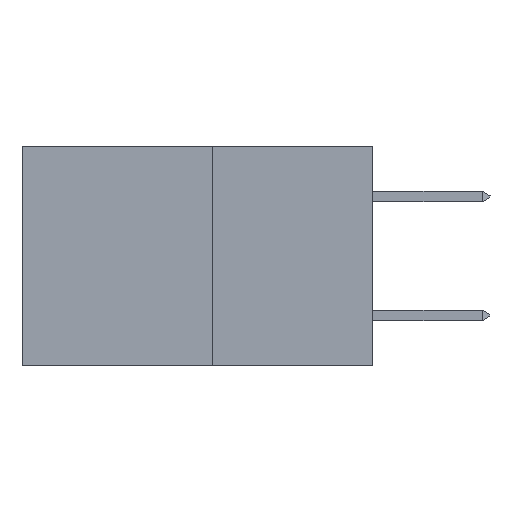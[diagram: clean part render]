
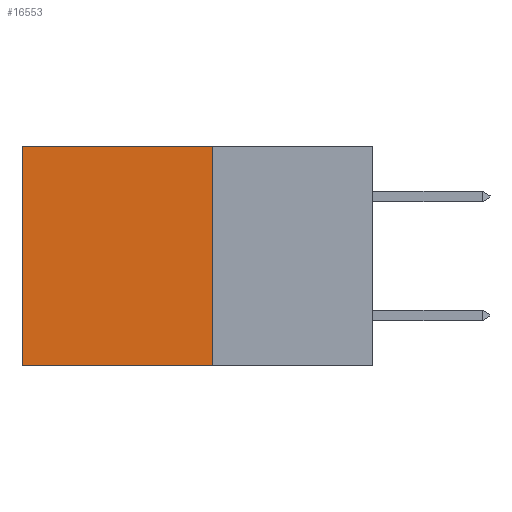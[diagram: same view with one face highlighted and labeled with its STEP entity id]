
A CAD part, left-side view. The second image highlights one B-rep face of the part: STEP entity #16553.
In plain terms, the highlighted planar face has unit normal (-1, 0, 0).
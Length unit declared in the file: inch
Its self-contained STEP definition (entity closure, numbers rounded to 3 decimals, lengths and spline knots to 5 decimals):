
#2171 = CARTESIAN_POINT ( 'NONE',  ( 0.277, 0.27, 0. ) ) ;
#2743 = VERTEX_POINT ( 'NONE', #21457 ) ;
#3335 = LINE ( 'NONE', #29948, #29181 ) ;
#3987 = VECTOR ( 'NONE', #9623, 39.37008 ) ;
#4703 = VECTOR ( 'NONE', #7975, 39.37008 ) ;
#4783 = LINE ( 'NONE', #24999, #3987 ) ;
#4809 = VERTEX_POINT ( 'NONE', #19418 ) ;
#5365 = CARTESIAN_POINT ( 'NONE',  ( 0.277, 0.59, -0.37 ) ) ;
#6470 = ORIENTED_EDGE ( 'NONE', *, *, #17992, .T. ) ;
#7503 = VERTEX_POINT ( 'NONE', #2171 ) ;
#7975 = DIRECTION ( 'NONE',  ( 0., 0., -1. ) ) ;
#9475 = DIRECTION ( 'NONE',  ( 1., 0., 0. ) ) ;
#9519 = ORIENTED_EDGE ( 'NONE', *, *, #11198, .T. ) ;
#9623 = DIRECTION ( 'NONE',  ( 0., 0., -1. ) ) ;
#11198 = EDGE_CURVE ( 'NONE', #11613, #2743, #12356, .T. ) ;
#11613 = VERTEX_POINT ( 'NONE', #27595 ) ;
#12356 = LINE ( 'NONE', #5365, #4703 ) ;
#14869 = EDGE_LOOP ( 'NONE', ( #9519, #22660, #16639, #6470 ) ) ;
#15389 = AXIS2_PLACEMENT_3D ( 'NONE', #22327, #9475, #27559 ) ;
#16553 = ADVANCED_FACE ( 'NONE', ( #24858 ), #17136, .F. ) ;
#16639 = ORIENTED_EDGE ( 'NONE', *, *, #29217, .F. ) ;
#17136 = PLANE ( 'NONE',  #15389 ) ;
#17992 = EDGE_CURVE ( 'NONE', #7503, #11613, #3335, .T. ) ;
#19418 = CARTESIAN_POINT ( 'NONE',  ( 0.277, 0.27, -0.37 ) ) ;
#20380 = EDGE_CURVE ( 'NONE', #4809, #2743, #24997, .T. ) ;
#21457 = CARTESIAN_POINT ( 'NONE',  ( 0.277, 0.59, -0.37 ) ) ;
#22158 = CARTESIAN_POINT ( 'NONE',  ( 0.277, 0.27, -0.37 ) ) ;
#22327 = CARTESIAN_POINT ( 'NONE',  ( 0.277, 0.27, -0.37 ) ) ;
#22660 = ORIENTED_EDGE ( 'NONE', *, *, #20380, .F. ) ;
#24858 = FACE_OUTER_BOUND ( 'NONE', #14869, .T. ) ;
#24877 = DIRECTION ( 'NONE',  ( 0., 1., 0. ) ) ;
#24901 = DIRECTION ( 'NONE',  ( 0., 1., 0. ) ) ;
#24997 = LINE ( 'NONE', #22158, #31029 ) ;
#24999 = CARTESIAN_POINT ( 'NONE',  ( 0.277, 0.27, -0.37 ) ) ;
#27559 = DIRECTION ( 'NONE',  ( 0., 0., -1. ) ) ;
#27595 = CARTESIAN_POINT ( 'NONE',  ( 0.277, 0.59, 0. ) ) ;
#29181 = VECTOR ( 'NONE', #24877, 39.37008 ) ;
#29217 = EDGE_CURVE ( 'NONE', #7503, #4809, #4783, .T. ) ;
#29948 = CARTESIAN_POINT ( 'NONE',  ( 0.277, 0.27, 0. ) ) ;
#31029 = VECTOR ( 'NONE', #24901, 39.37008 ) ;
